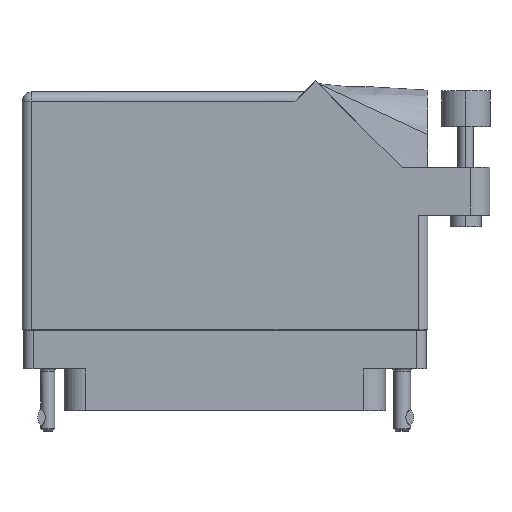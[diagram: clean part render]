
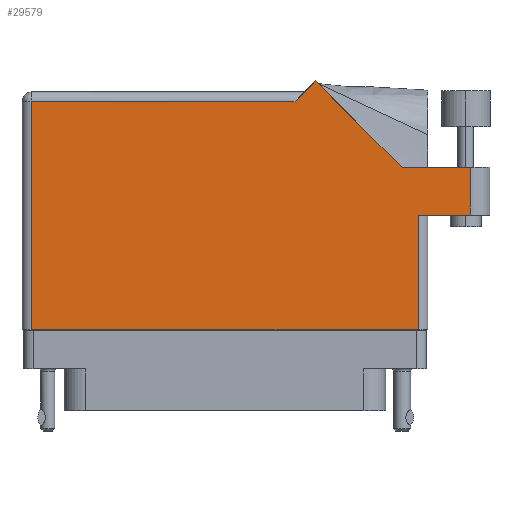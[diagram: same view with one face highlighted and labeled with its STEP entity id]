
A CAD part, front view. The second image highlights one B-rep face of the part: STEP entity #29579.
In plain terms, the highlighted face is planar.
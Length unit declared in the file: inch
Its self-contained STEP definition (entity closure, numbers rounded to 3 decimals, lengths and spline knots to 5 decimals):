
#132 = EDGE_CURVE ( 'NONE', #46075, #56483, #16845, .T. ) ;
#826 = PLANE ( 'NONE',  #4145 ) ;
#913 = LINE ( 'NONE', #57471, #49821 ) ;
#4012 = ORIENTED_EDGE ( 'NONE', *, *, #132, .T. ) ;
#4145 = AXIS2_PLACEMENT_3D ( 'NONE', #18492, #15048, #37963 ) ;
#4951 = EDGE_CURVE ( 'NONE', #20662, #11077, #26044, .T. ) ;
#6408 = EDGE_CURVE ( 'NONE', #22440, #20662, #10536, .T. ) ;
#6784 = CARTESIAN_POINT ( 'NONE',  ( 1.581, 0.944, 0.455 ) ) ;
#7085 = LINE ( 'NONE', #6784, #10221 ) ;
#7112 = DIRECTION ( 'NONE',  ( 0., 1., 0. ) ) ;
#7444 = VERTEX_POINT ( 'NONE', #17790 ) ;
#7529 = CARTESIAN_POINT ( 'NONE',  ( 1.244, 0.637, 0.455 ) ) ;
#7989 = VECTOR ( 'NONE', #7112, 39.37008 ) ;
#8041 = ORIENTED_EDGE ( 'NONE', *, *, #6408, .T. ) ;
#8419 = CARTESIAN_POINT ( 'NONE',  ( -1.306, -0.1, 0.455 ) ) ;
#8497 = EDGE_CURVE ( 'NONE', #23350, #7444, #11802, .T. ) ;
#10221 = VECTOR ( 'NONE', #11726, 39.37008 ) ;
#10536 = LINE ( 'NONE', #48262, #49489 ) ;
#11077 = VERTEX_POINT ( 'NONE', #48546 ) ;
#11726 = DIRECTION ( 'NONE',  ( 0., 1., 0. ) ) ;
#11802 = LINE ( 'NONE', #36247, #55488 ) ;
#12051 = CARTESIAN_POINT ( 'NONE',  ( 1.244, 0.637, 0.455 ) ) ;
#14151 = FACE_OUTER_BOUND ( 'NONE', #51723, .T. ) ;
#15048 = DIRECTION ( 'NONE',  ( 0., 0., -1. ) ) ;
#16096 = EDGE_CURVE ( 'NONE', #11077, #46075, #21332, .T. ) ;
#16673 = VECTOR ( 'NONE', #60182, 39.37008 ) ;
#16845 = LINE ( 'NONE', #27662, #30027 ) ;
#17659 = ORIENTED_EDGE ( 'NONE', *, *, #21702, .T. ) ;
#17790 = CARTESIAN_POINT ( 'NONE',  ( 0.58371, 1.50071, 0.455 ) ) ;
#18492 = CARTESIAN_POINT ( 'NONE',  ( -1.306, 1.43, 0.455 ) ) ;
#20350 = VERTEX_POINT ( 'NONE', #40421 ) ;
#20662 = VERTEX_POINT ( 'NONE', #34352 ) ;
#21332 = LINE ( 'NONE', #12051, #7989 ) ;
#21702 = EDGE_CURVE ( 'NONE', #60086, #23350, #39137, .T. ) ;
#22440 = VERTEX_POINT ( 'NONE', #42571 ) ;
#22709 = DIRECTION ( 'NONE',  ( 1., 0., 0. ) ) ;
#22754 = LINE ( 'NONE', #42531, #16673 ) ;
#23350 = VERTEX_POINT ( 'NONE', #47835 ) ;
#23513 = ORIENTED_EDGE ( 'NONE', *, *, #31618, .T. ) ;
#23724 = ORIENTED_EDGE ( 'NONE', *, *, #8497, .T. ) ;
#25210 = CARTESIAN_POINT ( 'NONE',  ( 1.706, 0.944, 0.455 ) ) ;
#26044 = LINE ( 'NONE', #8419, #45289 ) ;
#27662 = CARTESIAN_POINT ( 'NONE',  ( 1.306, 0.637, 0.455 ) ) ;
#29579 = ADVANCED_FACE ( 'NONE', ( #14151 ), #826, .F. ) ;
#30027 = VECTOR ( 'NONE', #22709, 39.37008 ) ;
#31618 = EDGE_CURVE ( 'NONE', #56483, #60086, #7085, .T. ) ;
#31691 = ORIENTED_EDGE ( 'NONE', *, *, #16096, .T. ) ;
#34005 = CARTESIAN_POINT ( 'NONE',  ( 1.581, 0.637, 0.455 ) ) ;
#34007 = DIRECTION ( 'NONE',  ( -1., 0., 0. ) ) ;
#34352 = CARTESIAN_POINT ( 'NONE',  ( -1.244, -0.1, 0.455 ) ) ;
#34540 = EDGE_CURVE ( 'NONE', #20350, #22440, #913, .T. ) ;
#36247 = CARTESIAN_POINT ( 'NONE',  ( 1.14042, 0.944, 0.455 ) ) ;
#37963 = DIRECTION ( 'NONE',  ( -1., 0., 0. ) ) ;
#38484 = CARTESIAN_POINT ( 'NONE',  ( 1.581, 0.944, 0.455 ) ) ;
#39009 = EDGE_CURVE ( 'NONE', #7444, #20350, #22754, .T. ) ;
#39080 = ORIENTED_EDGE ( 'NONE', *, *, #34540, .T. ) ;
#39137 = LINE ( 'NONE', #25210, #60684 ) ;
#40421 = CARTESIAN_POINT ( 'NONE',  ( 0.451, 1.368, 0.455 ) ) ;
#41914 = ORIENTED_EDGE ( 'NONE', *, *, #4951, .T. ) ;
#42531 = CARTESIAN_POINT ( 'NONE',  ( 0.513, 1.43, 0.455 ) ) ;
#42571 = CARTESIAN_POINT ( 'NONE',  ( -1.244, 1.368, 0.455 ) ) ;
#45289 = VECTOR ( 'NONE', #46140, 39.37008 ) ;
#46075 = VERTEX_POINT ( 'NONE', #7529 ) ;
#46140 = DIRECTION ( 'NONE',  ( 1., 0., 0. ) ) ;
#47835 = CARTESIAN_POINT ( 'NONE',  ( 1.14042, 0.944, 0.455 ) ) ;
#48262 = CARTESIAN_POINT ( 'NONE',  ( -1.244, -0.1, 0.455 ) ) ;
#48546 = CARTESIAN_POINT ( 'NONE',  ( 1.244, -0.1, 0.455 ) ) ;
#49489 = VECTOR ( 'NONE', #58450, 39.37008 ) ;
#49704 = ORIENTED_EDGE ( 'NONE', *, *, #39009, .T. ) ;
#49821 = VECTOR ( 'NONE', #34007, 39.37008 ) ;
#49831 = DIRECTION ( 'NONE',  ( -0.707, 0.707, 0. ) ) ;
#51723 = EDGE_LOOP ( 'NONE', ( #4012, #23513, #17659, #23724, #49704, #39080, #8041, #41914, #31691 ) ) ;
#55488 = VECTOR ( 'NONE', #49831, 39.37008 ) ;
#56483 = VERTEX_POINT ( 'NONE', #34005 ) ;
#57471 = CARTESIAN_POINT ( 'NONE',  ( -1.306, 1.368, 0.455 ) ) ;
#57983 = DIRECTION ( 'NONE',  ( -1., 0., 0. ) ) ;
#58450 = DIRECTION ( 'NONE',  ( 0., -1., 0. ) ) ;
#60086 = VERTEX_POINT ( 'NONE', #38484 ) ;
#60182 = DIRECTION ( 'NONE',  ( -0.707, -0.707, 0. ) ) ;
#60684 = VECTOR ( 'NONE', #57983, 39.37008 ) ;
